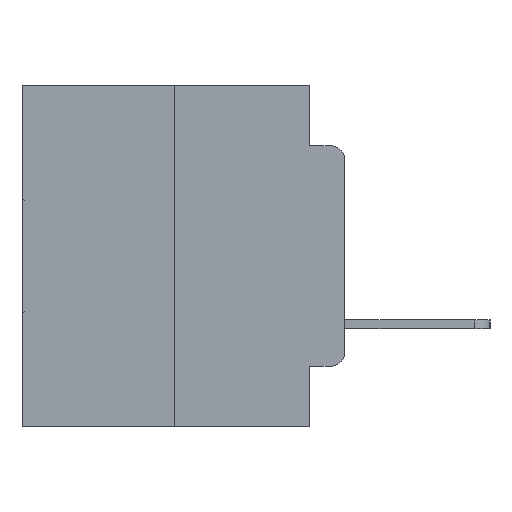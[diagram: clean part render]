
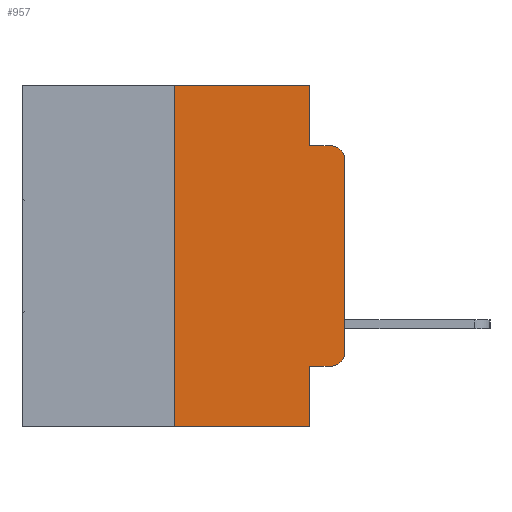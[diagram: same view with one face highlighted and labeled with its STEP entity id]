
A CAD part, left-side view. The second image highlights one B-rep face of the part: STEP entity #957.
In plain terms, the highlighted planar face has unit normal (-1, 0, 0).
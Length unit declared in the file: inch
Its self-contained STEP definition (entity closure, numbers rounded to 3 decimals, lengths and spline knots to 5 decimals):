
#59 = DIRECTION ( 'NONE',  ( 0., -1., 0. ) ) ;
#477 = VECTOR ( 'NONE', #9103, 39.37008 ) ;
#674 = ORIENTED_EDGE ( 'NONE', *, *, #7786, .T. ) ;
#706 = ORIENTED_EDGE ( 'NONE', *, *, #5990, .T. ) ;
#787 = VECTOR ( 'NONE', #14287, 39.37008 ) ;
#921 = ORIENTED_EDGE ( 'NONE', *, *, #25049, .F. ) ;
#957 = ADVANCED_FACE ( 'NONE', ( #17148 ), #26644, .F. ) ;
#961 = LINE ( 'NONE', #27447, #6503 ) ;
#996 = ORIENTED_EDGE ( 'NONE', *, *, #29201, .F. ) ;
#1026 = ORIENTED_EDGE ( 'NONE', *, *, #29439, .F. ) ;
#1493 = ORIENTED_EDGE ( 'NONE', *, *, #27564, .F. ) ;
#1602 = ORIENTED_EDGE ( 'NONE', *, *, #10273, .T. ) ;
#1662 = ORIENTED_EDGE ( 'NONE', *, *, #20757, .F. ) ;
#1817 = CARTESIAN_POINT ( 'NONE',  ( 0., 0.051, -0.4115 ) ) ;
#1861 = ORIENTED_EDGE ( 'NONE', *, *, #12084, .T. ) ;
#2034 = ORIENTED_EDGE ( 'NONE', *, *, #21148, .T. ) ;
#2420 = CARTESIAN_POINT ( 'NONE',  ( 0., 0., -0.1085 ) ) ;
#2529 = CARTESIAN_POINT ( 'NONE',  ( 0., 0.051, -0.4115 ) ) ;
#2822 = CARTESIAN_POINT ( 'NONE',  ( 0., 0.473, 0. ) ) ;
#3054 = CARTESIAN_POINT ( 'NONE',  ( 0., 0.25, 0. ) ) ;
#3196 = AXIS2_PLACEMENT_3D ( 'NONE', #7220, #22993, #9509 ) ;
#4042 = CARTESIAN_POINT ( 'NONE',  ( 0., 0.051, -0.0885 ) ) ;
#4160 = VERTEX_POINT ( 'NONE', #26969 ) ;
#5126 = VECTOR ( 'NONE', #12927, 39.37008 ) ;
#5301 = VECTOR ( 'NONE', #18806, 39.37008 ) ;
#5990 = EDGE_CURVE ( 'NONE', #14519, #28601, #10715, .T. ) ;
#6503 = VECTOR ( 'NONE', #59, 39.37008 ) ;
#6556 = CARTESIAN_POINT ( 'NONE',  ( 0., 0.02, -0.0885 ) ) ;
#7220 = CARTESIAN_POINT ( 'NONE',  ( 0., 0.02, -0.3915 ) ) ;
#7679 = LINE ( 'NONE', #8710, #24243 ) ;
#7786 = EDGE_CURVE ( 'NONE', #15954, #14519, #21175, .T. ) ;
#8521 = DIRECTION ( 'NONE',  ( 1., 0., 0. ) ) ;
#8689 = CARTESIAN_POINT ( 'NONE',  ( 0., 0.02, -0.1085 ) ) ;
#8710 = CARTESIAN_POINT ( 'NONE',  ( 0., 0.051, 0. ) ) ;
#9103 = DIRECTION ( 'NONE',  ( 0., 0., -1. ) ) ;
#9509 = DIRECTION ( 'NONE',  ( 0., 0., -1. ) ) ;
#9586 = CARTESIAN_POINT ( 'NONE',  ( 0., 0., 0. ) ) ;
#10273 = EDGE_CURVE ( 'NONE', #27723, #4160, #961, .T. ) ;
#10715 = CIRCLE ( 'NONE', #11826, 0.02 ) ;
#10977 = LINE ( 'NONE', #2529, #27537 ) ;
#10979 = DIRECTION ( 'NONE',  ( 0., 0., -1. ) ) ;
#11316 = VERTEX_POINT ( 'NONE', #13210 ) ;
#11347 = VERTEX_POINT ( 'NONE', #1817 ) ;
#11826 = AXIS2_PLACEMENT_3D ( 'NONE', #8689, #24457, #10979 ) ;
#11879 = DIRECTION ( 'NONE',  ( 0., 0., 1. ) ) ;
#12007 = CARTESIAN_POINT ( 'NONE',  ( 0., 0.25, 0. ) ) ;
#12084 = EDGE_CURVE ( 'NONE', #11347, #22917, #10977, .T. ) ;
#12927 = DIRECTION ( 'NONE',  ( 0., -1., 0. ) ) ;
#13210 = CARTESIAN_POINT ( 'NONE',  ( 0., 0.051, 0. ) ) ;
#14287 = DIRECTION ( 'NONE',  ( 0., 0., 1. ) ) ;
#14478 = EDGE_LOOP ( 'NONE', ( #674, #706, #921, #996, #1026, #1493, #1602, #1662, #1861, #2034 ) ) ;
#14519 = VERTEX_POINT ( 'NONE', #2420 ) ;
#15878 = CARTESIAN_POINT ( 'NONE',  ( 0., 0.051, 0. ) ) ;
#15954 = VERTEX_POINT ( 'NONE', #24302 ) ;
#17148 = FACE_OUTER_BOUND ( 'NONE', #14478, .T. ) ;
#17261 = LINE ( 'NONE', #26410, #5126 ) ;
#18760 = CARTESIAN_POINT ( 'NONE',  ( 0., 0.473, 0. ) ) ;
#18806 = DIRECTION ( 'NONE',  ( 0., -1., 0. ) ) ;
#19127 = LINE ( 'NONE', #12007, #787 ) ;
#20379 = DIRECTION ( 'NONE',  ( 0., 0., -1. ) ) ;
#20757 = EDGE_CURVE ( 'NONE', #11347, #4160, #24100, .T. ) ;
#20973 = CARTESIAN_POINT ( 'NONE',  ( 0., 0.02, -0.4115 ) ) ;
#21148 = EDGE_CURVE ( 'NONE', #22917, #15954, #25474, .T. ) ;
#21175 = LINE ( 'NONE', #9586, #27134 ) ;
#21553 = CARTESIAN_POINT ( 'NONE',  ( 0., 0.25, -0.5 ) ) ;
#22312 = DIRECTION ( 'NONE',  ( 0., 0., -1. ) ) ;
#22917 = VERTEX_POINT ( 'NONE', #20973 ) ;
#22993 = DIRECTION ( 'NONE',  ( -1., 0., 0. ) ) ;
#24100 = LINE ( 'NONE', #15878, #477 ) ;
#24243 = VECTOR ( 'NONE', #22312, 39.37008 ) ;
#24302 = CARTESIAN_POINT ( 'NONE',  ( 0., 0., -0.3915 ) ) ;
#24457 = DIRECTION ( 'NONE',  ( -1., 0., 0. ) ) ;
#25049 = EDGE_CURVE ( 'NONE', #25671, #28601, #17261, .T. ) ;
#25179 = DIRECTION ( 'NONE',  ( 0., -1., 0. ) ) ;
#25474 = CIRCLE ( 'NONE', #3196, 0.02 ) ;
#25671 = VERTEX_POINT ( 'NONE', #4042 ) ;
#26410 = CARTESIAN_POINT ( 'NONE',  ( 0., 0.051, -0.0885 ) ) ;
#26644 = PLANE ( 'NONE',  #28882 ) ;
#26681 = VERTEX_POINT ( 'NONE', #3054 ) ;
#26969 = CARTESIAN_POINT ( 'NONE',  ( 0., 0.051, -0.5 ) ) ;
#27134 = VECTOR ( 'NONE', #11879, 39.37008 ) ;
#27447 = CARTESIAN_POINT ( 'NONE',  ( 0., 0.473, -0.5 ) ) ;
#27537 = VECTOR ( 'NONE', #25179, 39.37008 ) ;
#27564 = EDGE_CURVE ( 'NONE', #27723, #26681, #19127, .T. ) ;
#27723 = VERTEX_POINT ( 'NONE', #21553 ) ;
#27962 = LINE ( 'NONE', #2822, #5301 ) ;
#28601 = VERTEX_POINT ( 'NONE', #6556 ) ;
#28882 = AXIS2_PLACEMENT_3D ( 'NONE', #18760, #8521, #20379 ) ;
#29201 = EDGE_CURVE ( 'NONE', #11316, #25671, #7679, .T. ) ;
#29439 = EDGE_CURVE ( 'NONE', #26681, #11316, #27962, .T. ) ;
